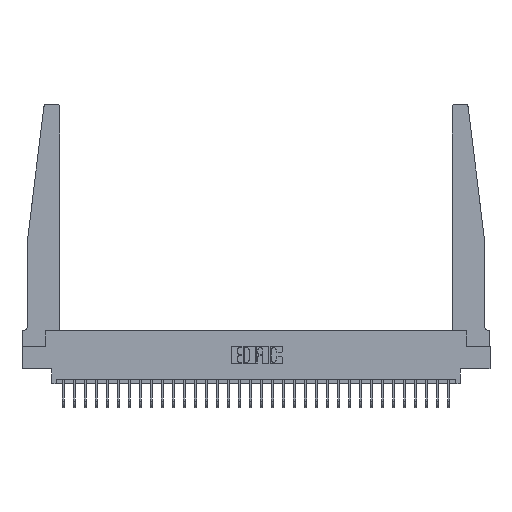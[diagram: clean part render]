
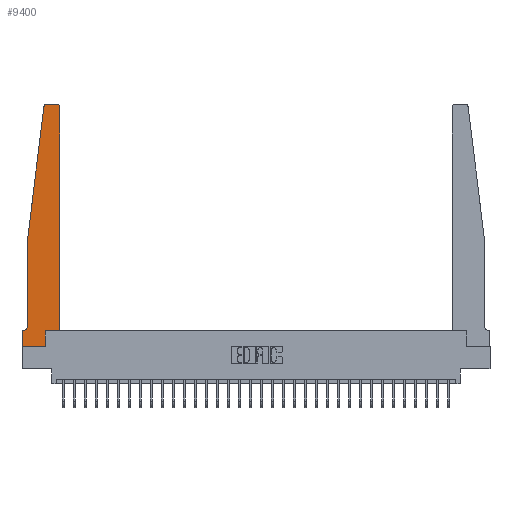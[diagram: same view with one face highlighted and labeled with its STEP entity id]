
A CAD part, top view. The second image highlights one B-rep face of the part: STEP entity #9400.
In plain terms, the highlighted planar face has unit normal (0, 0, 1).
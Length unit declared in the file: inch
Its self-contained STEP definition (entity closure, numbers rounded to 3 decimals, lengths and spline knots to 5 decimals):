
#43 = LINE ( 'NONE', #19605, #22156 ) ;
#300 = ORIENTED_EDGE ( 'NONE', *, *, #24562, .T. ) ;
#564 = ORIENTED_EDGE ( 'NONE', *, *, #3179, .T. ) ;
#863 = DIRECTION ( 'NONE',  ( -1., 0., 0. ) ) ;
#2191 = VERTEX_POINT ( 'NONE', #15777 ) ;
#2877 = EDGE_CURVE ( 'NONE', #21287, #14283, #12935, .T. ) ;
#3179 = EDGE_CURVE ( 'NONE', #13036, #22666, #43, .T. ) ;
#3559 = FACE_OUTER_BOUND ( 'NONE', #28146, .T. ) ;
#3749 = LINE ( 'NONE', #30461, #25848 ) ;
#4168 = EDGE_CURVE ( 'NONE', #2191, #9488, #27813, .T. ) ;
#4647 = DIRECTION ( 'NONE',  ( -0.122, -0.992, 0. ) ) ;
#5390 = LINE ( 'NONE', #15391, #18686 ) ;
#6602 = DIRECTION ( 'NONE',  ( 1., 0., 0. ) ) ;
#6686 = DIRECTION ( 'NONE',  ( 0., 0., 1. ) ) ;
#6707 = AXIS2_PLACEMENT_3D ( 'NONE', #21784, #26137, #28209 ) ;
#6763 = CARTESIAN_POINT ( 'NONE',  ( 0.425, 0.18, 0.37 ) ) ;
#6917 = EDGE_CURVE ( 'NONE', #18903, #27235, #18859, .T. ) ;
#7417 = DIRECTION ( 'NONE',  ( 0., 0., 1. ) ) ;
#8397 = DIRECTION ( 'NONE',  ( -1., 0., 0. ) ) ;
#8677 = ORIENTED_EDGE ( 'NONE', *, *, #27105, .T. ) ;
#8774 = ORIENTED_EDGE ( 'NONE', *, *, #2877, .T. ) ;
#9400 = ADVANCED_FACE ( 'NONE', ( #3559 ), #9802, .T. ) ;
#9488 = VERTEX_POINT ( 'NONE', #11345 ) ;
#9802 = PLANE ( 'NONE',  #14684 ) ;
#10099 = CARTESIAN_POINT ( 'NONE',  ( 0.425, 2.72, 0.37 ) ) ;
#10222 = DIRECTION ( 'NONE',  ( 0., -1., 0. ) ) ;
#10522 = AXIS2_PLACEMENT_3D ( 'NONE', #30968, #13764, #6602 ) ;
#10737 = CARTESIAN_POINT ( 'NONE',  ( 0.065, 0.1875, 0.37 ) ) ;
#11324 = CARTESIAN_POINT ( 'NONE',  ( 0.395, 2.72, 0.37 ) ) ;
#11345 = CARTESIAN_POINT ( 'NONE',  ( 0.24675, 2.72367, 0.37 ) ) ;
#11380 = EDGE_CURVE ( 'NONE', #22666, #21287, #27535, .T. ) ;
#11382 = CARTESIAN_POINT ( 'NONE',  ( 0.425, 0.18, 0.37 ) ) ;
#11444 = DIRECTION ( 'NONE',  ( 1., 0., 0. ) ) ;
#11483 = VERTEX_POINT ( 'NONE', #12842 ) ;
#12842 = CARTESIAN_POINT ( 'NONE',  ( 0., 0., 0.37 ) ) ;
#12935 = LINE ( 'NONE', #10737, #23172 ) ;
#13036 = VERTEX_POINT ( 'NONE', #18861 ) ;
#13070 = EDGE_CURVE ( 'NONE', #27235, #30207, #14083, .T. ) ;
#13429 = DIRECTION ( 'NONE',  ( 0., 1., 0. ) ) ;
#13764 = DIRECTION ( 'NONE',  ( 0., 0., 1. ) ) ;
#14083 = LINE ( 'NONE', #18389, #14532 ) ;
#14283 = VERTEX_POINT ( 'NONE', #23534 ) ;
#14532 = VECTOR ( 'NONE', #25710, 39.37008 ) ;
#14684 = AXIS2_PLACEMENT_3D ( 'NONE', #29212, #7417, #17267 ) ;
#15391 = CARTESIAN_POINT ( 'NONE',  ( 0.25, 2.75, 0.37 ) ) ;
#15705 = VECTOR ( 'NONE', #31340, 39.37008 ) ;
#15777 = CARTESIAN_POINT ( 'NONE',  ( 0.27653, 2.75, 0.37 ) ) ;
#16411 = CARTESIAN_POINT ( 'NONE',  ( 0.065, 1.25, 0.37 ) ) ;
#16458 = DIRECTION ( 'NONE',  ( 1., 0., 0. ) ) ;
#16727 = CARTESIAN_POINT ( 'NONE',  ( 0.065, 0.2375, 0.37 ) ) ;
#17053 = ORIENTED_EDGE ( 'NONE', *, *, #18734, .T. ) ;
#17110 = VECTOR ( 'NONE', #11444, 39.37008 ) ;
#17267 = DIRECTION ( 'NONE',  ( 1., 0., 0. ) ) ;
#18389 = CARTESIAN_POINT ( 'NONE',  ( 0.425, 0.18, 0.37 ) ) ;
#18606 = ORIENTED_EDGE ( 'NONE', *, *, #30809, .T. ) ;
#18642 = ORIENTED_EDGE ( 'NONE', *, *, #27786, .T. ) ;
#18686 = VECTOR ( 'NONE', #8397, 39.37008 ) ;
#18734 = EDGE_CURVE ( 'NONE', #30207, #22151, #29616, .T. ) ;
#18859 = LINE ( 'NONE', #6763, #25119 ) ;
#18861 = CARTESIAN_POINT ( 'NONE',  ( 0.065, 1.25, 0.37 ) ) ;
#18903 = VERTEX_POINT ( 'NONE', #27193 ) ;
#19380 = CARTESIAN_POINT ( 'NONE',  ( 0., 0., 0.37 ) ) ;
#19605 = CARTESIAN_POINT ( 'NONE',  ( 0.065, 1.25, 0.37 ) ) ;
#21287 = VERTEX_POINT ( 'NONE', #24935 ) ;
#21409 = VECTOR ( 'NONE', #4647, 39.37008 ) ;
#21602 = CARTESIAN_POINT ( 'NONE',  ( 0., 0., 0.37 ) ) ;
#21784 = CARTESIAN_POINT ( 'NONE',  ( 0.015, 0.2375, 0.37 ) ) ;
#22151 = VERTEX_POINT ( 'NONE', #25857 ) ;
#22156 = VECTOR ( 'NONE', #10222, 39.37008 ) ;
#22660 = ORIENTED_EDGE ( 'NONE', *, *, #6917, .T. ) ;
#22666 = VERTEX_POINT ( 'NONE', #16727 ) ;
#23172 = VECTOR ( 'NONE', #863, 39.37008 ) ;
#23534 = CARTESIAN_POINT ( 'NONE',  ( 0., 0.1875, 0.37 ) ) ;
#23701 = CARTESIAN_POINT ( 'NONE',  ( 0.2605, 0., 0.37 ) ) ;
#24028 = LINE ( 'NONE', #19380, #15705 ) ;
#24562 = EDGE_CURVE ( 'NONE', #22151, #2191, #5390, .T. ) ;
#24627 = ORIENTED_EDGE ( 'NONE', *, *, #13070, .T. ) ;
#24662 = ORIENTED_EDGE ( 'NONE', *, *, #11380, .T. ) ;
#24935 = CARTESIAN_POINT ( 'NONE',  ( 0.015, 0.1875, 0.37 ) ) ;
#25119 = VECTOR ( 'NONE', #16458, 39.37008 ) ;
#25130 = EDGE_CURVE ( 'NONE', #11483, #26322, #29089, .T. ) ;
#25158 = ORIENTED_EDGE ( 'NONE', *, *, #4168, .T. ) ;
#25710 = DIRECTION ( 'NONE',  ( 0., 1., 0. ) ) ;
#25848 = VECTOR ( 'NONE', #13429, 39.37008 ) ;
#25857 = CARTESIAN_POINT ( 'NONE',  ( 0.395, 2.75, 0.37 ) ) ;
#26137 = DIRECTION ( 'NONE',  ( 0., 0., -1. ) ) ;
#26322 = VERTEX_POINT ( 'NONE', #23701 ) ;
#26440 = LINE ( 'NONE', #16411, #21409 ) ;
#27105 = EDGE_CURVE ( 'NONE', #26322, #18903, #3749, .T. ) ;
#27193 = CARTESIAN_POINT ( 'NONE',  ( 0.2605, 0.18, 0.37 ) ) ;
#27235 = VERTEX_POINT ( 'NONE', #11382 ) ;
#27535 = CIRCLE ( 'NONE', #6707, 0.05 ) ;
#27786 = EDGE_CURVE ( 'NONE', #14283, #11483, #24028, .T. ) ;
#27813 = CIRCLE ( 'NONE', #10522, 0.03 ) ;
#28146 = EDGE_LOOP ( 'NONE', ( #300, #25158, #18606, #564, #24662, #8774, #18642, #28926, #8677, #22660, #24627, #17053 ) ) ;
#28209 = DIRECTION ( 'NONE',  ( -1., 0., 0. ) ) ;
#28926 = ORIENTED_EDGE ( 'NONE', *, *, #25130, .T. ) ;
#29089 = LINE ( 'NONE', #21602, #17110 ) ;
#29129 = AXIS2_PLACEMENT_3D ( 'NONE', #11324, #6686, #31038 ) ;
#29212 = CARTESIAN_POINT ( 'NONE',  ( 0., 0.1875, 0.37 ) ) ;
#29616 = CIRCLE ( 'NONE', #29129, 0.03 ) ;
#30207 = VERTEX_POINT ( 'NONE', #10099 ) ;
#30461 = CARTESIAN_POINT ( 'NONE',  ( 0.2605, 0.18, 0.37 ) ) ;
#30809 = EDGE_CURVE ( 'NONE', #9488, #13036, #26440, .T. ) ;
#30968 = CARTESIAN_POINT ( 'NONE',  ( 0.27653, 2.72, 0.37 ) ) ;
#31038 = DIRECTION ( 'NONE',  ( 1., 0., 0. ) ) ;
#31340 = DIRECTION ( 'NONE',  ( 0., -1., 0. ) ) ;
